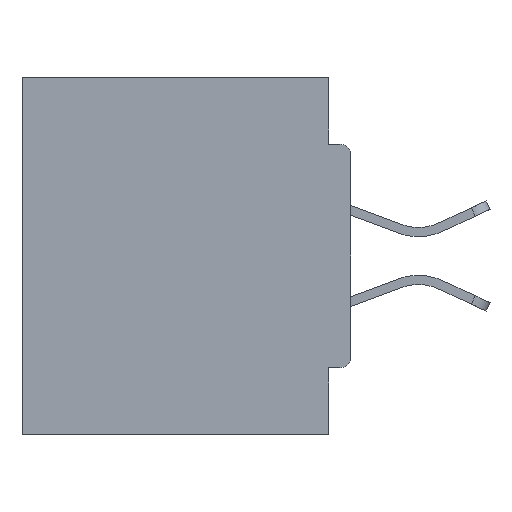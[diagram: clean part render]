
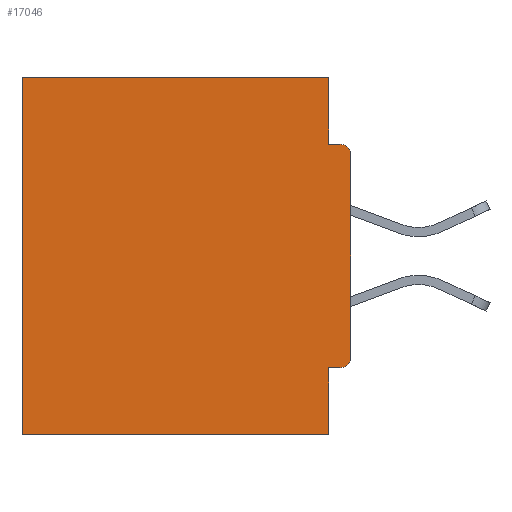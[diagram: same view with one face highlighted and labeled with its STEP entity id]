
A CAD part, left-side view. The second image highlights one B-rep face of the part: STEP entity #17046.
In plain terms, the highlighted planar face has unit normal (-1, 0, 0).
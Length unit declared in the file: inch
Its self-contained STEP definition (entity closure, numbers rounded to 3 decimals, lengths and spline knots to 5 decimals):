
#1394 = CIRCLE ( 'NONE', #3646, 0.015 ) ;
#2420 = LINE ( 'NONE', #32038, #8629 ) ;
#2765 = DIRECTION ( 'NONE',  ( 0., 1., 0. ) ) ;
#2987 = CARTESIAN_POINT ( 'NONE',  ( 0.298, 0.46, -0.5 ) ) ;
#2991 = VECTOR ( 'NONE', #22179, 39.37008 ) ;
#3115 = LINE ( 'NONE', #3297, #13659 ) ;
#3297 = CARTESIAN_POINT ( 'NONE',  ( 0.298, 0., -0.4065 ) ) ;
#3406 = CARTESIAN_POINT ( 'NONE',  ( 0.298, 0.031, -0.5 ) ) ;
#3646 = AXIS2_PLACEMENT_3D ( 'NONE', #10571, #16722, #34641 ) ;
#4911 = EDGE_CURVE ( 'NONE', #19502, #5466, #16715, .T. ) ;
#5125 = DIRECTION ( 'NONE',  ( 1., 0., 0. ) ) ;
#5466 = VERTEX_POINT ( 'NONE', #30146 ) ;
#5606 = DIRECTION ( 'NONE',  ( 0., 1., 0. ) ) ;
#6639 = VECTOR ( 'NONE', #39314, 39.37008 ) ;
#7147 = ORIENTED_EDGE ( 'NONE', *, *, #37344, .T. ) ;
#8101 = VERTEX_POINT ( 'NONE', #15589 ) ;
#8629 = VECTOR ( 'NONE', #19894, 39.37008 ) ;
#9292 = EDGE_CURVE ( 'NONE', #38459, #36265, #26438, .T. ) ;
#9939 = LINE ( 'NONE', #10105, #35289 ) ;
#10105 = CARTESIAN_POINT ( 'NONE',  ( 0.298, 0.031, -0.5 ) ) ;
#10262 = VERTEX_POINT ( 'NONE', #25537 ) ;
#10438 = FACE_OUTER_BOUND ( 'NONE', #29674, .T. ) ;
#10450 = CARTESIAN_POINT ( 'NONE',  ( 0.298, 0.015, -0.1085 ) ) ;
#10464 = VECTOR ( 'NONE', #21168, 39.37008 ) ;
#10571 = CARTESIAN_POINT ( 'NONE',  ( 0.298, 0.015, -0.3915 ) ) ;
#11193 = ORIENTED_EDGE ( 'NONE', *, *, #27066, .T. ) ;
#11852 = EDGE_CURVE ( 'NONE', #20496, #38459, #9939, .T. ) ;
#13659 = VECTOR ( 'NONE', #2765, 39.37008 ) ;
#13849 = VECTOR ( 'NONE', #5606, 39.37008 ) ;
#15097 = ORIENTED_EDGE ( 'NONE', *, *, #9292, .F. ) ;
#15118 = ORIENTED_EDGE ( 'NONE', *, *, #25199, .T. ) ;
#15589 = CARTESIAN_POINT ( 'NONE',  ( 0.298, 0.031, -0.0935 ) ) ;
#15691 = EDGE_CURVE ( 'NONE', #36955, #8101, #18578, .T. ) ;
#16715 = LINE ( 'NONE', #23662, #6639 ) ;
#16722 = DIRECTION ( 'NONE',  ( -1., 0., 0. ) ) ;
#17046 = ADVANCED_FACE ( 'NONE', ( #10438 ), #26515, .F. ) ;
#17274 = DIRECTION ( 'NONE',  ( 0., 0., -1. ) ) ;
#17889 = VERTEX_POINT ( 'NONE', #28881 ) ;
#18578 = LINE ( 'NONE', #3406, #10464 ) ;
#19502 = VERTEX_POINT ( 'NONE', #32106 ) ;
#19894 = DIRECTION ( 'NONE',  ( 0., -1., 0. ) ) ;
#19942 = DIRECTION ( 'NONE',  ( 0., 0., -1. ) ) ;
#20496 = VERTEX_POINT ( 'NONE', #28727 ) ;
#20597 = AXIS2_PLACEMENT_3D ( 'NONE', #10450, #37962, #19942 ) ;
#20651 = DIRECTION ( 'NONE',  ( 0., 0., -1. ) ) ;
#20785 = ORIENTED_EDGE ( 'NONE', *, *, #35015, .F. ) ;
#21168 = DIRECTION ( 'NONE',  ( 0., 0., -1. ) ) ;
#22179 = DIRECTION ( 'NONE',  ( 0., 1., 0. ) ) ;
#22475 = LINE ( 'NONE', #36327, #13849 ) ;
#23662 = CARTESIAN_POINT ( 'NONE',  ( 0.298, 0., 0. ) ) ;
#24100 = EDGE_CURVE ( 'NONE', #8101, #24566, #2420, .T. ) ;
#24566 = VERTEX_POINT ( 'NONE', #31476 ) ;
#25199 = EDGE_CURVE ( 'NONE', #10262, #5466, #1394, .T. ) ;
#25282 = CARTESIAN_POINT ( 'NONE',  ( 0.298, 0., -0.5 ) ) ;
#25346 = ORIENTED_EDGE ( 'NONE', *, *, #4911, .F. ) ;
#25537 = CARTESIAN_POINT ( 'NONE',  ( 0.298, 0.015, -0.4065 ) ) ;
#26438 = LINE ( 'NONE', #25282, #2991 ) ;
#26515 = PLANE ( 'NONE',  #28530 ) ;
#27066 = EDGE_CURVE ( 'NONE', #17889, #36265, #37395, .T. ) ;
#27849 = ORIENTED_EDGE ( 'NONE', *, *, #15691, .F. ) ;
#28350 = VECTOR ( 'NONE', #20651, 39.37008 ) ;
#28530 = AXIS2_PLACEMENT_3D ( 'NONE', #38523, #5125, #17274 ) ;
#28727 = CARTESIAN_POINT ( 'NONE',  ( 0.298, 0.031, -0.4065 ) ) ;
#28881 = CARTESIAN_POINT ( 'NONE',  ( 0.298, 0.46, 0. ) ) ;
#29116 = CARTESIAN_POINT ( 'NONE',  ( 0.298, 0.031, 0. ) ) ;
#29674 = EDGE_LOOP ( 'NONE', ( #7147, #29693, #27849, #35838, #11193, #15097, #35645, #20785, #15118, #25346 ) ) ;
#29693 = ORIENTED_EDGE ( 'NONE', *, *, #24100, .F. ) ;
#30146 = CARTESIAN_POINT ( 'NONE',  ( 0.298, 0., -0.3915 ) ) ;
#31476 = CARTESIAN_POINT ( 'NONE',  ( 0.298, 0.015, -0.0935 ) ) ;
#31487 = DIRECTION ( 'NONE',  ( 0., 0., -1. ) ) ;
#32038 = CARTESIAN_POINT ( 'NONE',  ( 0.298, 0., -0.0935 ) ) ;
#32106 = CARTESIAN_POINT ( 'NONE',  ( 0.298, 0., -0.1085 ) ) ;
#33867 = CARTESIAN_POINT ( 'NONE',  ( 0.298, 0.031, -0.5 ) ) ;
#34498 = CIRCLE ( 'NONE', #20597, 0.015 ) ;
#34641 = DIRECTION ( 'NONE',  ( 0., 0., -1. ) ) ;
#35015 = EDGE_CURVE ( 'NONE', #10262, #20496, #3115, .T. ) ;
#35289 = VECTOR ( 'NONE', #31487, 39.37008 ) ;
#35351 = CARTESIAN_POINT ( 'NONE',  ( 0.298, 0.46, 0. ) ) ;
#35645 = ORIENTED_EDGE ( 'NONE', *, *, #11852, .F. ) ;
#35838 = ORIENTED_EDGE ( 'NONE', *, *, #37747, .T. ) ;
#36265 = VERTEX_POINT ( 'NONE', #2987 ) ;
#36327 = CARTESIAN_POINT ( 'NONE',  ( 0.298, 0., 0. ) ) ;
#36955 = VERTEX_POINT ( 'NONE', #29116 ) ;
#37344 = EDGE_CURVE ( 'NONE', #19502, #24566, #34498, .T. ) ;
#37395 = LINE ( 'NONE', #35351, #28350 ) ;
#37747 = EDGE_CURVE ( 'NONE', #36955, #17889, #22475, .T. ) ;
#37962 = DIRECTION ( 'NONE',  ( -1., 0., 0. ) ) ;
#38459 = VERTEX_POINT ( 'NONE', #33867 ) ;
#38523 = CARTESIAN_POINT ( 'NONE',  ( 0.298, 0., 0. ) ) ;
#39314 = DIRECTION ( 'NONE',  ( 0., 0., -1. ) ) ;
